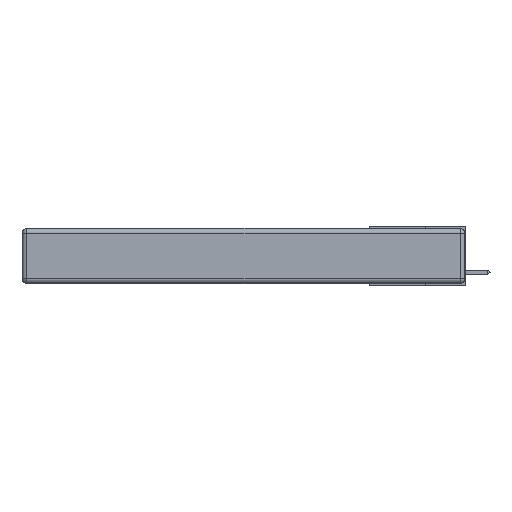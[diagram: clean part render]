
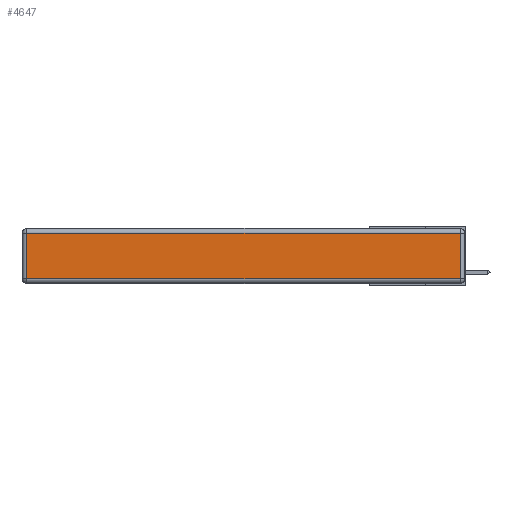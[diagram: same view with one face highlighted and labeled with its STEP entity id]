
A CAD part, left-side view. The second image highlights one B-rep face of the part: STEP entity #4647.
In plain terms, the highlighted planar face has unit normal (-1, 0, 0).
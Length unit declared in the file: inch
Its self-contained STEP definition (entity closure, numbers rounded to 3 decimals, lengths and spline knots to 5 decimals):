
#288 = CARTESIAN_POINT ( 'NONE',  ( 0., 2.72, -0.03 ) ) ;
#418 = DIRECTION ( 'NONE',  ( -1., 0., 0. ) ) ;
#2593 = EDGE_CURVE ( 'NONE', #13136, #11167, #5898, .T. ) ;
#3383 = CARTESIAN_POINT ( 'NONE',  ( 0., 0.03, -0.313 ) ) ;
#3665 = DIRECTION ( 'NONE',  ( 0., 0., 1. ) ) ;
#3934 = CARTESIAN_POINT ( 'NONE',  ( 0., 0., -0.343 ) ) ;
#4146 = EDGE_LOOP ( 'NONE', ( #23479, #10154, #4717, #22459 ) ) ;
#4647 = ADVANCED_FACE ( 'NONE', ( #10900 ), #5664, .T. ) ;
#4717 = ORIENTED_EDGE ( 'NONE', *, *, #2593, .T. ) ;
#5223 = AXIS2_PLACEMENT_3D ( 'NONE', #3934, #418, #20197 ) ;
#5463 = CARTESIAN_POINT ( 'NONE',  ( 0., 0.03, -0.343 ) ) ;
#5471 = CARTESIAN_POINT ( 'NONE',  ( 0., 2.72, -0.343 ) ) ;
#5664 = PLANE ( 'NONE',  #5223 ) ;
#5898 = LINE ( 'NONE', #17157, #16690 ) ;
#8046 = CARTESIAN_POINT ( 'NONE',  ( 0., 0.03, -0.03 ) ) ;
#8612 = EDGE_CURVE ( 'NONE', #11167, #14248, #15696, .T. ) ;
#9192 = VECTOR ( 'NONE', #3665, 39.37008 ) ;
#9377 = EDGE_CURVE ( 'NONE', #14248, #15226, #9956, .T. ) ;
#9731 = CARTESIAN_POINT ( 'NONE',  ( 0., 2.72, -0.313 ) ) ;
#9956 = LINE ( 'NONE', #18767, #16207 ) ;
#10154 = ORIENTED_EDGE ( 'NONE', *, *, #19951, .T. ) ;
#10900 = FACE_OUTER_BOUND ( 'NONE', #4146, .T. ) ;
#11167 = VERTEX_POINT ( 'NONE', #288 ) ;
#12815 = DIRECTION ( 'NONE',  ( 0., 0., -1. ) ) ;
#13136 = VERTEX_POINT ( 'NONE', #8046 ) ;
#14248 = VERTEX_POINT ( 'NONE', #9731 ) ;
#15226 = VERTEX_POINT ( 'NONE', #3383 ) ;
#15696 = LINE ( 'NONE', #5471, #19655 ) ;
#16207 = VECTOR ( 'NONE', #16864, 39.37008 ) ;
#16690 = VECTOR ( 'NONE', #22751, 39.37008 ) ;
#16864 = DIRECTION ( 'NONE',  ( 0., -1., 0. ) ) ;
#17157 = CARTESIAN_POINT ( 'NONE',  ( 0., 2.75, -0.03 ) ) ;
#18767 = CARTESIAN_POINT ( 'NONE',  ( 0., 0., -0.313 ) ) ;
#19655 = VECTOR ( 'NONE', #12815, 39.37008 ) ;
#19951 = EDGE_CURVE ( 'NONE', #15226, #13136, #22001, .T. ) ;
#20197 = DIRECTION ( 'NONE',  ( 0., 0., 1. ) ) ;
#22001 = LINE ( 'NONE', #5463, #9192 ) ;
#22459 = ORIENTED_EDGE ( 'NONE', *, *, #8612, .T. ) ;
#22751 = DIRECTION ( 'NONE',  ( 0., 1., 0. ) ) ;
#23479 = ORIENTED_EDGE ( 'NONE', *, *, #9377, .T. ) ;
